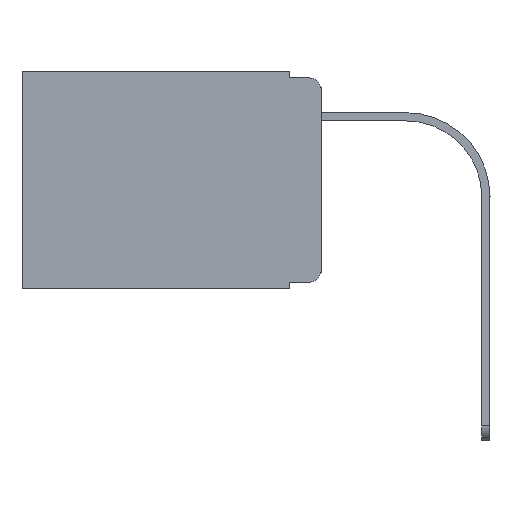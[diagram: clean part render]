
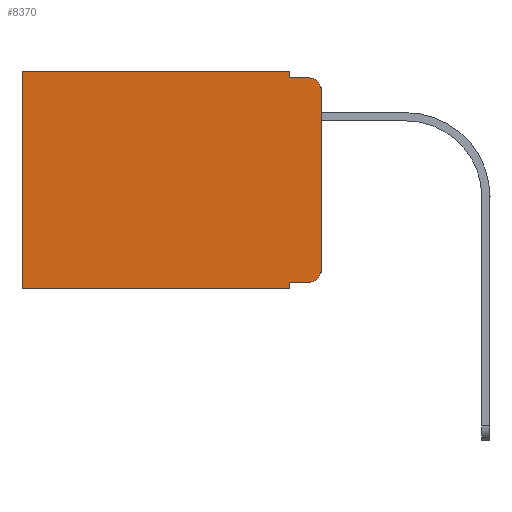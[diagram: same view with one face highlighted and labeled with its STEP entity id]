
A CAD part, left-side view. The second image highlights one B-rep face of the part: STEP entity #8370.
In plain terms, the highlighted planar face has unit normal (-1, 0, 0).
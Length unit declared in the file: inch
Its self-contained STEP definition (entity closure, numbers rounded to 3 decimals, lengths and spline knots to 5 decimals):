
#18 = EDGE_CURVE ( 'NONE', #14400, #9611, #14401, .T. ) ;
#721 = DIRECTION ( 'NONE',  ( -1., 0., 0. ) ) ;
#829 = DIRECTION ( 'NONE',  ( 0., 0., -1. ) ) ;
#909 = CARTESIAN_POINT ( 'NONE',  ( 0.298, 0.02, -0.333 ) ) ;
#1185 = DIRECTION ( 'NONE',  ( 0., 0., -1. ) ) ;
#1276 = CIRCLE ( 'NONE', #18440, 0.02 ) ;
#1494 = CARTESIAN_POINT ( 'NONE',  ( 0.298, 0.473, 0. ) ) ;
#1725 = AXIS2_PLACEMENT_3D ( 'NONE', #3670, #4064, #2279 ) ;
#2080 = EDGE_CURVE ( 'NONE', #15301, #19605, #10162, .T. ) ;
#2112 = EDGE_LOOP ( 'NONE', ( #19077, #17881, #11189, #14828, #3905, #13326, #13783, #5457, #4372, #16290 ) ) ;
#2279 = DIRECTION ( 'NONE',  ( 0., 0., -1. ) ) ;
#2408 = VECTOR ( 'NONE', #10072, 39.37008 ) ;
#2535 = EDGE_CURVE ( 'NONE', #3944, #12987, #17721, .T. ) ;
#2568 = FACE_OUTER_BOUND ( 'NONE', #2112, .T. ) ;
#2569 = DIRECTION ( 'NONE',  ( 0., 1., 0. ) ) ;
#2762 = EDGE_CURVE ( 'NONE', #11174, #9117, #6509, .T. ) ;
#2832 = EDGE_CURVE ( 'NONE', #9117, #12987, #11393, .T. ) ;
#3670 = CARTESIAN_POINT ( 'NONE',  ( 0.298, 0., 0. ) ) ;
#3744 = DIRECTION ( 'NONE',  ( 0., 0., -1. ) ) ;
#3905 = ORIENTED_EDGE ( 'NONE', *, *, #14726, .T. ) ;
#3944 = VERTEX_POINT ( 'NONE', #1494 ) ;
#3977 = CARTESIAN_POINT ( 'NONE',  ( 0.298, 0., -0.313 ) ) ;
#4064 = DIRECTION ( 'NONE',  ( 1., 0., 0. ) ) ;
#4372 = ORIENTED_EDGE ( 'NONE', *, *, #8164, .T. ) ;
#5457 = ORIENTED_EDGE ( 'NONE', *, *, #2762, .F. ) ;
#5528 = CARTESIAN_POINT ( 'NONE',  ( 0.298, 0., 0. ) ) ;
#6206 = VECTOR ( 'NONE', #1185, 39.37008 ) ;
#6509 = LINE ( 'NONE', #6604, #15476 ) ;
#6604 = CARTESIAN_POINT ( 'NONE',  ( 0.298, 0.051, 0. ) ) ;
#8020 = LINE ( 'NONE', #15735, #12508 ) ;
#8164 = EDGE_CURVE ( 'NONE', #11174, #18937, #8020, .T. ) ;
#8209 = DIRECTION ( 'NONE',  ( 0., 0., -1. ) ) ;
#8370 = ADVANCED_FACE ( 'NONE', ( #2568 ), #17716, .F. ) ;
#8860 = CARTESIAN_POINT ( 'NONE',  ( 0.298, 0.051, -0.01 ) ) ;
#9117 = VERTEX_POINT ( 'NONE', #13784 ) ;
#9268 = EDGE_CURVE ( 'NONE', #14400, #19605, #1276, .T. ) ;
#9297 = CARTESIAN_POINT ( 'NONE',  ( 0.298, 0.02, -0.313 ) ) ;
#9611 = VERTEX_POINT ( 'NONE', #3977 ) ;
#10072 = DIRECTION ( 'NONE',  ( 0., -1., 0. ) ) ;
#10162 = LINE ( 'NONE', #8860, #2408 ) ;
#10322 = VECTOR ( 'NONE', #8209, 39.37008 ) ;
#10682 = VECTOR ( 'NONE', #17489, 39.37008 ) ;
#10920 = DIRECTION ( 'NONE',  ( 0., -1., 0. ) ) ;
#11093 = CARTESIAN_POINT ( 'NONE',  ( 0.298, 0., -0.343 ) ) ;
#11174 = VERTEX_POINT ( 'NONE', #15110 ) ;
#11189 = ORIENTED_EDGE ( 'NONE', *, *, #2080, .F. ) ;
#11299 = CARTESIAN_POINT ( 'NONE',  ( 0.298, 0.051, 0. ) ) ;
#11393 = LINE ( 'NONE', #11093, #10682 ) ;
#12162 = CARTESIAN_POINT ( 'NONE',  ( 0.298, 0.051, 0. ) ) ;
#12508 = VECTOR ( 'NONE', #10920, 39.37008 ) ;
#12512 = LINE ( 'NONE', #11299, #10322 ) ;
#12914 = DIRECTION ( 'NONE',  ( 0., 0., -1. ) ) ;
#12987 = VERTEX_POINT ( 'NONE', #16264 ) ;
#13326 = ORIENTED_EDGE ( 'NONE', *, *, #2535, .T. ) ;
#13783 = ORIENTED_EDGE ( 'NONE', *, *, #2832, .F. ) ;
#13784 = CARTESIAN_POINT ( 'NONE',  ( 0.298, 0.051, -0.343 ) ) ;
#13977 = DIRECTION ( 'NONE',  ( -1., 0., 0. ) ) ;
#14376 = CARTESIAN_POINT ( 'NONE',  ( 0.298, 0.02, -0.03 ) ) ;
#14400 = VERTEX_POINT ( 'NONE', #18493 ) ;
#14401 = LINE ( 'NONE', #5528, #17646 ) ;
#14637 = CIRCLE ( 'NONE', #15595, 0.02 ) ;
#14720 = CARTESIAN_POINT ( 'NONE',  ( 0.298, 0., 0. ) ) ;
#14726 = EDGE_CURVE ( 'NONE', #18583, #3944, #18005, .T. ) ;
#14828 = ORIENTED_EDGE ( 'NONE', *, *, #15007, .F. ) ;
#15007 = EDGE_CURVE ( 'NONE', #18583, #15301, #12512, .T. ) ;
#15110 = CARTESIAN_POINT ( 'NONE',  ( 0.298, 0.051, -0.333 ) ) ;
#15301 = VERTEX_POINT ( 'NONE', #16691 ) ;
#15476 = VECTOR ( 'NONE', #3744, 39.37008 ) ;
#15595 = AXIS2_PLACEMENT_3D ( 'NONE', #9297, #13977, #18453 ) ;
#15735 = CARTESIAN_POINT ( 'NONE',  ( 0.298, 0.051, -0.333 ) ) ;
#16264 = CARTESIAN_POINT ( 'NONE',  ( 0.298, 0.473, -0.343 ) ) ;
#16290 = ORIENTED_EDGE ( 'NONE', *, *, #16373, .T. ) ;
#16373 = EDGE_CURVE ( 'NONE', #18937, #9611, #14637, .T. ) ;
#16691 = CARTESIAN_POINT ( 'NONE',  ( 0.298, 0.051, -0.01 ) ) ;
#17489 = DIRECTION ( 'NONE',  ( 0., 1., 0. ) ) ;
#17620 = CARTESIAN_POINT ( 'NONE',  ( 0.298, 0.473, 0. ) ) ;
#17646 = VECTOR ( 'NONE', #12914, 39.37008 ) ;
#17716 = PLANE ( 'NONE',  #1725 ) ;
#17721 = LINE ( 'NONE', #17620, #6206 ) ;
#17881 = ORIENTED_EDGE ( 'NONE', *, *, #9268, .T. ) ;
#17950 = VECTOR ( 'NONE', #2569, 39.37008 ) ;
#18005 = LINE ( 'NONE', #14720, #17950 ) ;
#18440 = AXIS2_PLACEMENT_3D ( 'NONE', #14376, #721, #829 ) ;
#18453 = DIRECTION ( 'NONE',  ( 0., 0., -1. ) ) ;
#18493 = CARTESIAN_POINT ( 'NONE',  ( 0.298, 0., -0.03 ) ) ;
#18583 = VERTEX_POINT ( 'NONE', #12162 ) ;
#18937 = VERTEX_POINT ( 'NONE', #909 ) ;
#18971 = CARTESIAN_POINT ( 'NONE',  ( 0.298, 0.02, -0.01 ) ) ;
#19077 = ORIENTED_EDGE ( 'NONE', *, *, #18, .F. ) ;
#19605 = VERTEX_POINT ( 'NONE', #18971 ) ;
